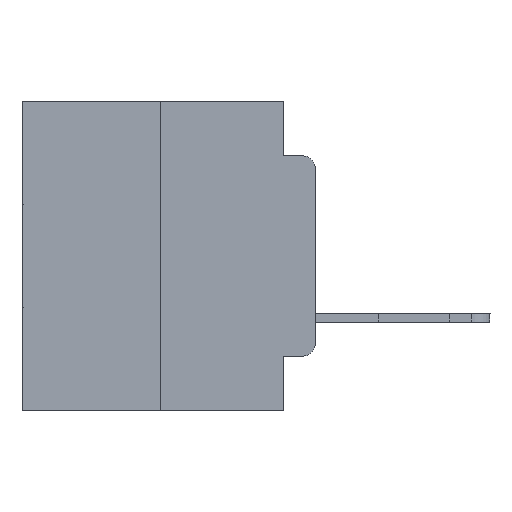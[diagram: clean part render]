
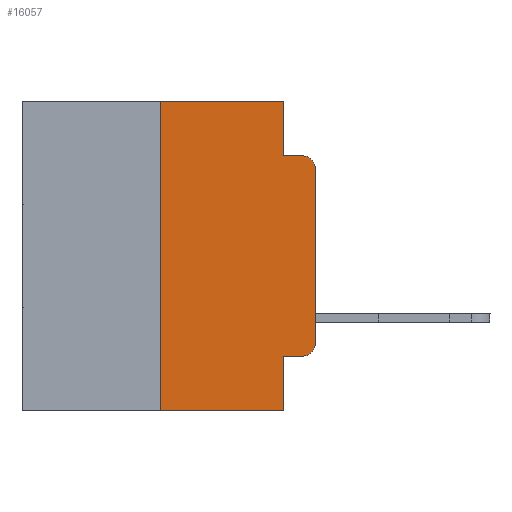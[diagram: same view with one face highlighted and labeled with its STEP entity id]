
A CAD part, left-side view. The second image highlights one B-rep face of the part: STEP entity #16057.
In plain terms, the highlighted planar face has unit normal (-1, 0, 0).
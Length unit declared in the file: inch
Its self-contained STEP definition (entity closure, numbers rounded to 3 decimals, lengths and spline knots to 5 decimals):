
#536 = ORIENTED_EDGE ( 'NONE', *, *, #1059, .F. ) ;
#1011 = EDGE_CURVE ( 'NONE', #25494, #5897, #7790, .T. ) ;
#1059 = EDGE_CURVE ( 'NONE', #9360, #15314, #17379, .T. ) ;
#1201 = VERTEX_POINT ( 'NONE', #8962 ) ;
#1403 = LINE ( 'NONE', #10382, #8680 ) ;
#1623 = EDGE_CURVE ( 'NONE', #11000, #1201, #17711, .T. ) ;
#1736 = DIRECTION ( 'NONE',  ( 0., 0., -1. ) ) ;
#2284 = CARTESIAN_POINT ( 'NONE',  ( 0., 0.02, -0.1085 ) ) ;
#2411 = EDGE_CURVE ( 'NONE', #24610, #15314, #2441, .T. ) ;
#2441 = CIRCLE ( 'NONE', #22188, 0.02 ) ;
#2904 = VERTEX_POINT ( 'NONE', #15499 ) ;
#3700 = DIRECTION ( 'NONE',  ( -1., 0., 0. ) ) ;
#3840 = CARTESIAN_POINT ( 'NONE',  ( 0., 0.051, -0.0885 ) ) ;
#4104 = VECTOR ( 'NONE', #15495, 39.37008 ) ;
#4780 = DIRECTION ( 'NONE',  ( -1., 0., 0. ) ) ;
#4786 = EDGE_LOOP ( 'NONE', ( #7729, #10069, #536, #18114, #15456, #22232, #12631, #8953, #19244, #5560 ) ) ;
#4857 = VERTEX_POINT ( 'NONE', #10445 ) ;
#4899 = CARTESIAN_POINT ( 'NONE',  ( 0., 0.051, -0.0885 ) ) ;
#5090 = CARTESIAN_POINT ( 'NONE',  ( 0., 0.02, -0.4115 ) ) ;
#5560 = ORIENTED_EDGE ( 'NONE', *, *, #1011, .T. ) ;
#5897 = VERTEX_POINT ( 'NONE', #24667 ) ;
#5970 = DIRECTION ( 'NONE',  ( 0., 0., 1. ) ) ;
#6230 = LINE ( 'NONE', #20064, #20989 ) ;
#7531 = DIRECTION ( 'NONE',  ( 0., -1., 0. ) ) ;
#7729 = ORIENTED_EDGE ( 'NONE', *, *, #19585, .T. ) ;
#7790 = CIRCLE ( 'NONE', #18600, 0.02 ) ;
#8129 = EDGE_CURVE ( 'NONE', #4857, #9360, #22965, .T. ) ;
#8483 = VERTEX_POINT ( 'NONE', #8641 ) ;
#8617 = EDGE_CURVE ( 'NONE', #2904, #8483, #18946, .T. ) ;
#8641 = CARTESIAN_POINT ( 'NONE',  ( 0., 0.051, -0.5 ) ) ;
#8680 = VECTOR ( 'NONE', #5970, 39.37008 ) ;
#8867 = EDGE_CURVE ( 'NONE', #1201, #4857, #24348, .T. ) ;
#8953 = ORIENTED_EDGE ( 'NONE', *, *, #8617, .F. ) ;
#8962 = CARTESIAN_POINT ( 'NONE',  ( 0., 0.25, 0. ) ) ;
#9282 = VECTOR ( 'NONE', #19948, 39.37008 ) ;
#9352 = EDGE_CURVE ( 'NONE', #2904, #25494, #6230, .T. ) ;
#9360 = VERTEX_POINT ( 'NONE', #4899 ) ;
#9701 = CARTESIAN_POINT ( 'NONE',  ( 0., 0.051, 0. ) ) ;
#10069 = ORIENTED_EDGE ( 'NONE', *, *, #2411, .T. ) ;
#10218 = VECTOR ( 'NONE', #16460, 39.37008 ) ;
#10382 = CARTESIAN_POINT ( 'NONE',  ( 0., 0., 0. ) ) ;
#10445 = CARTESIAN_POINT ( 'NONE',  ( 0., 0.051, 0. ) ) ;
#11000 = VERTEX_POINT ( 'NONE', #11538 ) ;
#11319 = CARTESIAN_POINT ( 'NONE',  ( 0., 0.02, -0.0885 ) ) ;
#11538 = CARTESIAN_POINT ( 'NONE',  ( 0., 0.25, -0.5 ) ) ;
#12631 = ORIENTED_EDGE ( 'NONE', *, *, #20482, .T. ) ;
#15213 = DIRECTION ( 'NONE',  ( 0., -1., 0. ) ) ;
#15314 = VERTEX_POINT ( 'NONE', #11319 ) ;
#15456 = ORIENTED_EDGE ( 'NONE', *, *, #8867, .F. ) ;
#15486 = PLANE ( 'NONE',  #20761 ) ;
#15495 = DIRECTION ( 'NONE',  ( 0., 0., 1. ) ) ;
#15499 = CARTESIAN_POINT ( 'NONE',  ( 0., 0.051, -0.4115 ) ) ;
#16057 = ADVANCED_FACE ( 'NONE', ( #24591 ), #15486, .F. ) ;
#16460 = DIRECTION ( 'NONE',  ( 0., 0., -1. ) ) ;
#17379 = LINE ( 'NONE', #3840, #19076 ) ;
#17661 = DIRECTION ( 'NONE',  ( 0., 0., -1. ) ) ;
#17711 = LINE ( 'NONE', #26967, #4104 ) ;
#18033 = CARTESIAN_POINT ( 'NONE',  ( 0., 0.473, 0. ) ) ;
#18114 = ORIENTED_EDGE ( 'NONE', *, *, #8129, .F. ) ;
#18397 = DIRECTION ( 'NONE',  ( 0., 0., -1. ) ) ;
#18600 = AXIS2_PLACEMENT_3D ( 'NONE', #26619, #3700, #17661 ) ;
#18728 = LINE ( 'NONE', #27700, #18997 ) ;
#18946 = LINE ( 'NONE', #27920, #10218 ) ;
#18997 = VECTOR ( 'NONE', #7531, 39.37008 ) ;
#19076 = VECTOR ( 'NONE', #22075, 39.37008 ) ;
#19244 = ORIENTED_EDGE ( 'NONE', *, *, #9352, .T. ) ;
#19585 = EDGE_CURVE ( 'NONE', #5897, #24610, #1403, .T. ) ;
#19948 = DIRECTION ( 'NONE',  ( 0., -1., 0. ) ) ;
#20064 = CARTESIAN_POINT ( 'NONE',  ( 0., 0.051, -0.4115 ) ) ;
#20482 = EDGE_CURVE ( 'NONE', #11000, #8483, #18728, .T. ) ;
#20624 = VECTOR ( 'NONE', #18397, 39.37008 ) ;
#20761 = AXIS2_PLACEMENT_3D ( 'NONE', #28731, #21969, #26518 ) ;
#20989 = VECTOR ( 'NONE', #15213, 39.37008 ) ;
#21969 = DIRECTION ( 'NONE',  ( 1., 0., 0. ) ) ;
#22075 = DIRECTION ( 'NONE',  ( 0., -1., 0. ) ) ;
#22188 = AXIS2_PLACEMENT_3D ( 'NONE', #2284, #4780, #1736 ) ;
#22232 = ORIENTED_EDGE ( 'NONE', *, *, #1623, .F. ) ;
#22965 = LINE ( 'NONE', #9701, #20624 ) ;
#24348 = LINE ( 'NONE', #18033, #9282 ) ;
#24591 = FACE_OUTER_BOUND ( 'NONE', #4786, .T. ) ;
#24610 = VERTEX_POINT ( 'NONE', #26975 ) ;
#24667 = CARTESIAN_POINT ( 'NONE',  ( 0., 0., -0.3915 ) ) ;
#25494 = VERTEX_POINT ( 'NONE', #5090 ) ;
#26518 = DIRECTION ( 'NONE',  ( 0., 0., -1. ) ) ;
#26619 = CARTESIAN_POINT ( 'NONE',  ( 0., 0.02, -0.3915 ) ) ;
#26967 = CARTESIAN_POINT ( 'NONE',  ( 0., 0.25, 0. ) ) ;
#26975 = CARTESIAN_POINT ( 'NONE',  ( 0., 0., -0.1085 ) ) ;
#27700 = CARTESIAN_POINT ( 'NONE',  ( 0., 0.473, -0.5 ) ) ;
#27920 = CARTESIAN_POINT ( 'NONE',  ( 0., 0.051, 0. ) ) ;
#28731 = CARTESIAN_POINT ( 'NONE',  ( 0., 0.473, 0. ) ) ;
